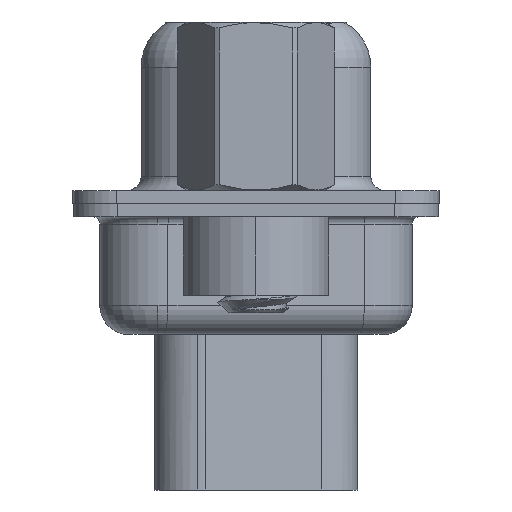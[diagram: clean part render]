
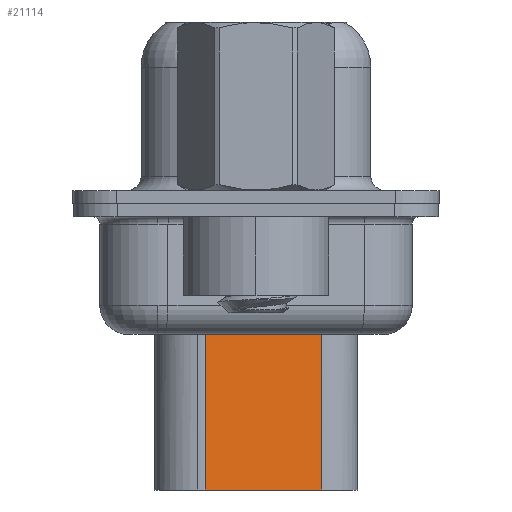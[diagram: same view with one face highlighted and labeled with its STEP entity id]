
A CAD part, left-side view. The second image highlights one B-rep face of the part: STEP entity #21114.
In plain terms, the highlighted planar face has unit normal (-0.985, -0.174, 0).
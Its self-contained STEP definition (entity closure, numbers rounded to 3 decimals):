
#865 = VECTOR ( 'NONE', #10738, 1000. ) ;
#1742 = CARTESIAN_POINT ( 'NONE',  ( 4.519, 1.74, -3.1 ) ) ;
#3330 = VECTOR ( 'NONE', #19766, 1000. ) ;
#4019 = VERTEX_POINT ( 'NONE', #16595 ) ;
#5887 = DIRECTION ( 'NONE',  ( 0.174, -0.985, 0. ) ) ;
#6029 = EDGE_CURVE ( 'NONE', #4019, #29152, #15151, .T. ) ;
#6807 = VECTOR ( 'NONE', #29511, 1000. ) ;
#8774 = ORIENTED_EDGE ( 'NONE', *, *, #29349, .T. ) ;
#10738 = DIRECTION ( 'NONE',  ( -0.174, 0.985, 0. ) ) ;
#11976 = AXIS2_PLACEMENT_3D ( 'NONE', #1742, #28880, #5887 ) ;
#12020 = CARTESIAN_POINT ( 'NONE',  ( 4.519, 1.74, -9.85 ) ) ;
#13342 = VERTEX_POINT ( 'NONE', #25662 ) ;
#13352 = FACE_OUTER_BOUND ( 'NONE', #28298, .T. ) ;
#13526 = CARTESIAN_POINT ( 'NONE',  ( 5.224, -2.26, -3.1 ) ) ;
#14995 = VECTOR ( 'NONE', #21445, 1000. ) ;
#15151 = LINE ( 'NONE', #17265, #865 ) ;
#16595 = CARTESIAN_POINT ( 'NONE',  ( 5.224, -2.26, -9.85 ) ) ;
#16723 = LINE ( 'NONE', #23721, #14995 ) ;
#17265 = CARTESIAN_POINT ( 'NONE',  ( 4.519, 1.74, -9.85 ) ) ;
#17305 = PLANE ( 'NONE',  #11976 ) ;
#17650 = CARTESIAN_POINT ( 'NONE',  ( 4.348, 2.709, -3.975 ) ) ;
#17669 = EDGE_CURVE ( 'NONE', #13342, #4019, #20208, .T. ) ;
#17761 = CARTESIAN_POINT ( 'NONE',  ( 4.519, 1.74, -3.975 ) ) ;
#19766 = DIRECTION ( 'NONE',  ( -0.174, 0.985, 0. ) ) ;
#20208 = LINE ( 'NONE', #13526, #6807 ) ;
#21114 = ADVANCED_FACE ( 'NONE', ( #13352 ), #17305, .T. ) ;
#21125 = VERTEX_POINT ( 'NONE', #17761 ) ;
#21445 = DIRECTION ( 'NONE',  ( 0., 0., -1. ) ) ;
#23721 = CARTESIAN_POINT ( 'NONE',  ( 4.519, 1.74, -3.1 ) ) ;
#23891 = ORIENTED_EDGE ( 'NONE', *, *, #17669, .F. ) ;
#25662 = CARTESIAN_POINT ( 'NONE',  ( 5.224, -2.26, -3.975 ) ) ;
#27118 = ORIENTED_EDGE ( 'NONE', *, *, #6029, .F. ) ;
#28298 = EDGE_LOOP ( 'NONE', ( #23891, #8774, #28302, #27118 ) ) ;
#28302 = ORIENTED_EDGE ( 'NONE', *, *, #28703, .T. ) ;
#28703 = EDGE_CURVE ( 'NONE', #21125, #29152, #16723, .T. ) ;
#28880 = DIRECTION ( 'NONE',  ( -0.985, -0.174, 0. ) ) ;
#29152 = VERTEX_POINT ( 'NONE', #12020 ) ;
#29231 = LINE ( 'NONE', #17650, #3330 ) ;
#29349 = EDGE_CURVE ( 'NONE', #13342, #21125, #29231, .T. ) ;
#29511 = DIRECTION ( 'NONE',  ( 0., 0., -1. ) ) ;
